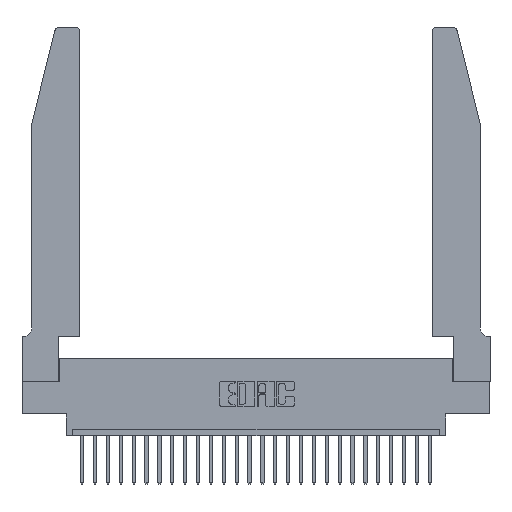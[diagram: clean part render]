
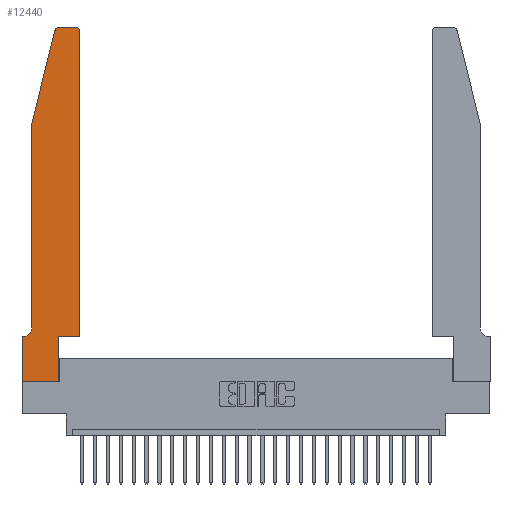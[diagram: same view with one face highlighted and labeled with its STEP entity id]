
A CAD part, top view. The second image highlights one B-rep face of the part: STEP entity #12440.
In plain terms, the highlighted planar face has unit normal (0, 0, 1).
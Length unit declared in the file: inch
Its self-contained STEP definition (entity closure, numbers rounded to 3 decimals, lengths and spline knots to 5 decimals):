
#127 = VERTEX_POINT ( 'NONE', #27602 ) ;
#187 = DIRECTION ( 'NONE',  ( 0., 0., 1. ) ) ;
#714 = LINE ( 'NONE', #14922, #27018 ) ;
#1169 = CIRCLE ( 'NONE', #10454, 0.03 ) ;
#1346 = ORIENTED_EDGE ( 'NONE', *, *, #8756, .T. ) ;
#1464 = LINE ( 'NONE', #27792, #20695 ) ;
#1538 = DIRECTION ( 'NONE',  ( 1., 0., 0. ) ) ;
#1613 = AXIS2_PLACEMENT_3D ( 'NONE', #15070, #6200, #8481 ) ;
#2302 = ORIENTED_EDGE ( 'NONE', *, *, #8204, .T. ) ;
#2819 = LINE ( 'NONE', #21803, #15338 ) ;
#2945 = CARTESIAN_POINT ( 'NONE',  ( 0., 0., 0.37 ) ) ;
#3330 = DIRECTION ( 'NONE',  ( 0., -1., 0. ) ) ;
#3368 = ORIENTED_EDGE ( 'NONE', *, *, #21793, .T. ) ;
#3519 = ORIENTED_EDGE ( 'NONE', *, *, #9844, .T. ) ;
#4676 = CARTESIAN_POINT ( 'NONE',  ( 0.2865, 0., 0.37 ) ) ;
#5340 = VECTOR ( 'NONE', #20868, 39.37008 ) ;
#5380 = CARTESIAN_POINT ( 'NONE',  ( 0.2865, 0.35, 0.37 ) ) ;
#5597 = DIRECTION ( 'NONE',  ( 0., 0., 1. ) ) ;
#6200 = DIRECTION ( 'NONE',  ( 0., 0., 1. ) ) ;
#6396 = DIRECTION ( 'NONE',  ( 1., 0., 0. ) ) ;
#6959 = VERTEX_POINT ( 'NONE', #4676 ) ;
#8146 = CARTESIAN_POINT ( 'NONE',  ( 0.0755, 0.35, 0.37 ) ) ;
#8204 = EDGE_CURVE ( 'NONE', #13028, #10990, #1169, .T. ) ;
#8418 = EDGE_CURVE ( 'NONE', #127, #13028, #2819, .T. ) ;
#8481 = DIRECTION ( 'NONE',  ( 1., 0., 0. ) ) ;
#8486 = CARTESIAN_POINT ( 'NONE',  ( 0.2605, 2.75, 0.37 ) ) ;
#8565 = DIRECTION ( 'NONE',  ( -0.239, -0.971, 0. ) ) ;
#8756 = EDGE_CURVE ( 'NONE', #17811, #20031, #26353, .T. ) ;
#8909 = CARTESIAN_POINT ( 'NONE',  ( 0.284, 2.72, 0.37 ) ) ;
#8928 = LINE ( 'NONE', #8486, #12320 ) ;
#9323 = CARTESIAN_POINT ( 'NONE',  ( 0., 0.35, 0.37 ) ) ;
#9328 = EDGE_CURVE ( 'NONE', #12464, #21529, #19276, .T. ) ;
#9405 = EDGE_CURVE ( 'NONE', #27472, #127, #714, .T. ) ;
#9547 = VECTOR ( 'NONE', #12383, 39.37008 ) ;
#9766 = DIRECTION ( 'NONE',  ( 0., 0., -1. ) ) ;
#9844 = EDGE_CURVE ( 'NONE', #21529, #12828, #12862, .T. ) ;
#10035 = EDGE_CURVE ( 'NONE', #12828, #6959, #20956, .T. ) ;
#10314 = CARTESIAN_POINT ( 'NONE',  ( 0.4205, 2.75, 0.37 ) ) ;
#10454 = AXIS2_PLACEMENT_3D ( 'NONE', #16384, #5597, #20686 ) ;
#10719 = ORIENTED_EDGE ( 'NONE', *, *, #20985, .T. ) ;
#10973 = CARTESIAN_POINT ( 'NONE',  ( 0.0755, 2., 0.37 ) ) ;
#10990 = VERTEX_POINT ( 'NONE', #10314 ) ;
#11172 = VECTOR ( 'NONE', #1538, 39.37008 ) ;
#12090 = CARTESIAN_POINT ( 'NONE',  ( 0.284, 2.75, 0.37 ) ) ;
#12092 = FACE_OUTER_BOUND ( 'NONE', #22489, .T. ) ;
#12320 = VECTOR ( 'NONE', #21626, 39.37008 ) ;
#12383 = DIRECTION ( 'NONE',  ( -1., 0., 0. ) ) ;
#12440 = ADVANCED_FACE ( 'NONE', ( #12092 ), #25665, .T. ) ;
#12464 = VERTEX_POINT ( 'NONE', #19358 ) ;
#12828 = VERTEX_POINT ( 'NONE', #2945 ) ;
#12862 = LINE ( 'NONE', #20781, #17588 ) ;
#13028 = VERTEX_POINT ( 'NONE', #25357 ) ;
#13767 = ORIENTED_EDGE ( 'NONE', *, *, #25143, .T. ) ;
#14096 = DIRECTION ( 'NONE',  ( -1., 0., 0. ) ) ;
#14303 = CARTESIAN_POINT ( 'NONE',  ( 0.25487, 2.72718, 0.37 ) ) ;
#14414 = DIRECTION ( 'NONE',  ( 0., -1., 0. ) ) ;
#14490 = CARTESIAN_POINT ( 'NONE',  ( 0., 0., 0.37 ) ) ;
#14531 = ORIENTED_EDGE ( 'NONE', *, *, #15215, .T. ) ;
#14922 = CARTESIAN_POINT ( 'NONE',  ( 0.4505, 0.35, 0.37 ) ) ;
#15070 = CARTESIAN_POINT ( 'NONE',  ( 0., 0.35, 0.37 ) ) ;
#15117 = AXIS2_PLACEMENT_3D ( 'NONE', #8909, #187, #15320 ) ;
#15137 = CIRCLE ( 'NONE', #18455, 0.07 ) ;
#15215 = EDGE_CURVE ( 'NONE', #20031, #12464, #15137, .T. ) ;
#15320 = DIRECTION ( 'NONE',  ( 1., 0., 0. ) ) ;
#15338 = VECTOR ( 'NONE', #24200, 39.37008 ) ;
#15356 = ORIENTED_EDGE ( 'NONE', *, *, #10035, .T. ) ;
#16384 = CARTESIAN_POINT ( 'NONE',  ( 0.4205, 2.72, 0.37 ) ) ;
#16829 = VERTEX_POINT ( 'NONE', #14303 ) ;
#17588 = VECTOR ( 'NONE', #14414, 39.37008 ) ;
#17811 = VERTEX_POINT ( 'NONE', #10973 ) ;
#17908 = CIRCLE ( 'NONE', #15117, 0.03 ) ;
#18088 = ORIENTED_EDGE ( 'NONE', *, *, #18837, .T. ) ;
#18407 = ORIENTED_EDGE ( 'NONE', *, *, #8418, .T. ) ;
#18455 = AXIS2_PLACEMENT_3D ( 'NONE', #20272, #9766, #14096 ) ;
#18837 = EDGE_CURVE ( 'NONE', #16829, #17811, #1464, .T. ) ;
#19276 = LINE ( 'NONE', #8146, #9547 ) ;
#19358 = CARTESIAN_POINT ( 'NONE',  ( 0.0055, 0.35, 0.37 ) ) ;
#19650 = ORIENTED_EDGE ( 'NONE', *, *, #9328, .T. ) ;
#19924 = CARTESIAN_POINT ( 'NONE',  ( 0.0755, 0.42, 0.37 ) ) ;
#20031 = VERTEX_POINT ( 'NONE', #19924 ) ;
#20272 = CARTESIAN_POINT ( 'NONE',  ( 0.0055, 0.42, 0.37 ) ) ;
#20683 = CARTESIAN_POINT ( 'NONE',  ( 0.2865, 0.35, 0.37 ) ) ;
#20686 = DIRECTION ( 'NONE',  ( 1., 0., 0. ) ) ;
#20691 = CARTESIAN_POINT ( 'NONE',  ( 0.0755, 2., 0.37 ) ) ;
#20695 = VECTOR ( 'NONE', #8565, 39.37008 ) ;
#20781 = CARTESIAN_POINT ( 'NONE',  ( 0., 0., 0.37 ) ) ;
#20868 = DIRECTION ( 'NONE',  ( 0., 1., 0. ) ) ;
#20956 = LINE ( 'NONE', #14490, #11172 ) ;
#20985 = EDGE_CURVE ( 'NONE', #25931, #16829, #17908, .T. ) ;
#21529 = VERTEX_POINT ( 'NONE', #9323 ) ;
#21626 = DIRECTION ( 'NONE',  ( -1., 0., 0. ) ) ;
#21793 = EDGE_CURVE ( 'NONE', #6959, #27472, #21850, .T. ) ;
#21803 = CARTESIAN_POINT ( 'NONE',  ( 0.4505, 0.35, 0.37 ) ) ;
#21850 = LINE ( 'NONE', #20683, #5340 ) ;
#22489 = EDGE_LOOP ( 'NONE', ( #13767, #10719, #18088, #1346, #14531, #19650, #3519, #15356, #3368, #25412, #18407, #2302 ) ) ;
#23985 = VECTOR ( 'NONE', #3330, 39.37008 ) ;
#24200 = DIRECTION ( 'NONE',  ( 0., 1., 0. ) ) ;
#25143 = EDGE_CURVE ( 'NONE', #10990, #25931, #8928, .T. ) ;
#25357 = CARTESIAN_POINT ( 'NONE',  ( 0.4505, 2.72, 0.37 ) ) ;
#25412 = ORIENTED_EDGE ( 'NONE', *, *, #9405, .T. ) ;
#25665 = PLANE ( 'NONE',  #1613 ) ;
#25931 = VERTEX_POINT ( 'NONE', #12090 ) ;
#26353 = LINE ( 'NONE', #20691, #23985 ) ;
#27018 = VECTOR ( 'NONE', #6396, 39.37008 ) ;
#27472 = VERTEX_POINT ( 'NONE', #5380 ) ;
#27602 = CARTESIAN_POINT ( 'NONE',  ( 0.4505, 0.35, 0.37 ) ) ;
#27792 = CARTESIAN_POINT ( 'NONE',  ( 0.0755, 2., 0.37 ) ) ;
